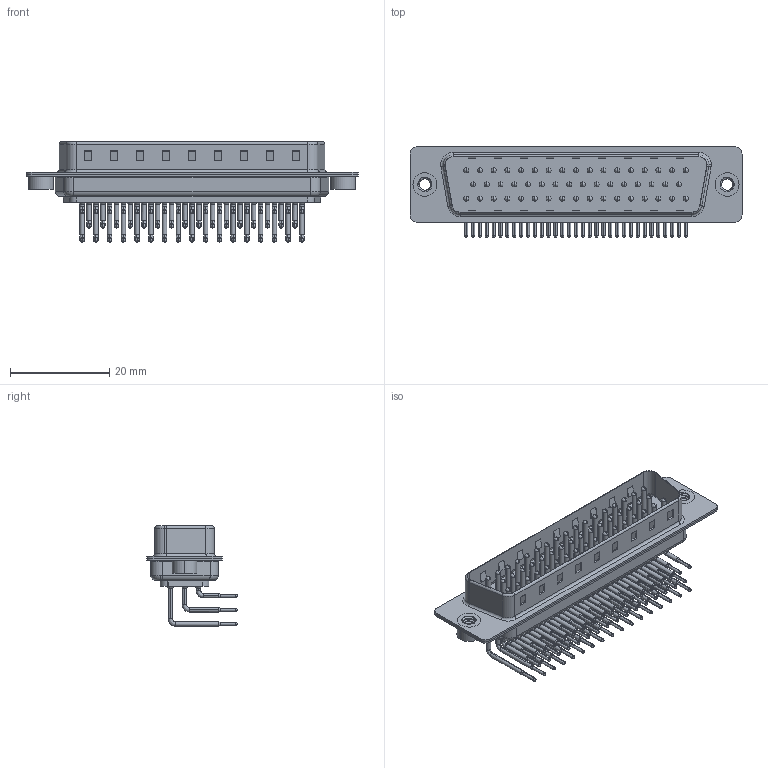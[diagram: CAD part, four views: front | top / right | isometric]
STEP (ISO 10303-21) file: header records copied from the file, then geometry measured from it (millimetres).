
FILE_DESCRIPTION (( 'STEP AP203' ), '1' );
FILE_NAME ('621-M50-260-LN2.STEP', '2018-09-25T11:36:07', ( '' ), ( '' ), 'SwSTEP 2.0', 'SolidWorks 2016', '' );
FILE_SCHEMA (( 'CONFIG_CONTROL_DESIGN' ));
Length unit declared in the file: millimetre
Products named in the file (8): 621-M50-260-LN2; 621M Housing_50 Contacts; 621M Shell Front_50 Contacts; 621M Shell Rear_50 Contacts; 621M Contact Row 1_50 Contacts; 621M Contact Row 2_50 Contacts; 621M Contact Row 3; 621M 4-40 Threaded Rivet
Assembly tree (55 placements, depth 2):
  621-M50-260-LN2
    621M Housing_50 Contacts
    621M Shell Front_50 Contacts
    621M Shell Rear_50 Contacts
    621M Contact Row 1_50 Contacts  x17
    621M Contact Row 2_50 Contacts  x16
    621M Contact Row 3  x17
    621M 4-40 Threaded Rivet  x2
Bounding box: 67 x 18.3 x 20.23 mm (x, y, z)
Volume: 4922.1 mm3; surface area: 12574.7 mm2
Topology: 55 solids, 55 shells, 5912 faces, 16593 edges, 10802 vertices
Faces by surface type: plane 3403, cylinder 1941, bspline 306, cone 206, torus 56
Entity records: 37159 total; most frequent: CARTESIAN_POINT 7509, DIRECTION 6061, ORIENTED_EDGE 5486, EDGE_CURVE 2743, AXIS2_PLACEMENT_3D 2245, VERTEX_POINT 1787, VECTOR 1571, LINE 1571
